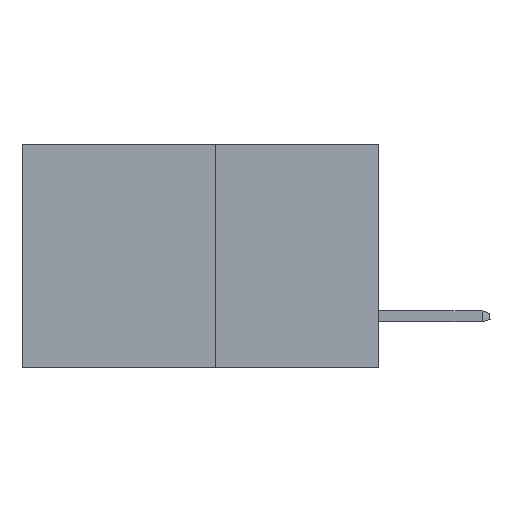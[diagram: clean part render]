
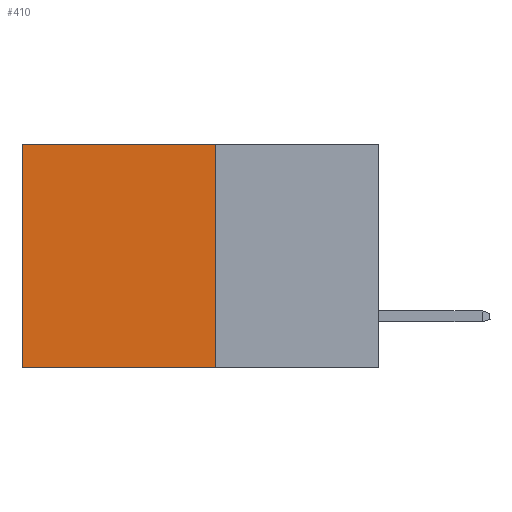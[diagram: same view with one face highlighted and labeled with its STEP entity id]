
A CAD part, left-side view. The second image highlights one B-rep face of the part: STEP entity #410.
In plain terms, the highlighted planar face has unit normal (-1, 0, 0).
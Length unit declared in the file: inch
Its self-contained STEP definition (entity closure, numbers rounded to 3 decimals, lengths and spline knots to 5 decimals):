
#97 = CARTESIAN_POINT ( 'NONE',  ( 0.277, 0.27, -0.37 ) ) ;
#312 = CARTESIAN_POINT ( 'NONE',  ( 0.277, 0.27, 0. ) ) ;
#410 = ADVANCED_FACE ( 'NONE', ( #12683 ), #1009, .F. ) ;
#500 = CARTESIAN_POINT ( 'NONE',  ( 0.277, 0.59, 0. ) ) ;
#1009 = PLANE ( 'NONE',  #9625 ) ;
#1131 = CARTESIAN_POINT ( 'NONE',  ( 0.277, 0.27, -0.37 ) ) ;
#1248 = CARTESIAN_POINT ( 'NONE',  ( 0.277, 0.27, -0.37 ) ) ;
#1303 = DIRECTION ( 'NONE',  ( 0., 0., -1. ) ) ;
#1486 = VECTOR ( 'NONE', #5163, 39.37008 ) ;
#2164 = DIRECTION ( 'NONE',  ( 0., 1., 0. ) ) ;
#3169 = VERTEX_POINT ( 'NONE', #9500 ) ;
#4032 = CARTESIAN_POINT ( 'NONE',  ( 0.277, 0.27, -0.37 ) ) ;
#4869 = LINE ( 'NONE', #1131, #10010 ) ;
#5163 = DIRECTION ( 'NONE',  ( 0., 1., 0. ) ) ;
#5440 = VERTEX_POINT ( 'NONE', #312 ) ;
#5594 = CARTESIAN_POINT ( 'NONE',  ( 0.277, 0.59, -0.37 ) ) ;
#5922 = LINE ( 'NONE', #5594, #8977 ) ;
#6097 = EDGE_CURVE ( 'NONE', #9296, #3169, #4869, .T. ) ;
#7016 = DIRECTION ( 'NONE',  ( 1., 0., 0. ) ) ;
#7064 = LINE ( 'NONE', #1248, #12114 ) ;
#7528 = VERTEX_POINT ( 'NONE', #500 ) ;
#7992 = EDGE_CURVE ( 'NONE', #5440, #9296, #7064, .T. ) ;
#8486 = EDGE_CURVE ( 'NONE', #5440, #7528, #9137, .T. ) ;
#8743 = EDGE_CURVE ( 'NONE', #7528, #3169, #5922, .T. ) ;
#8977 = VECTOR ( 'NONE', #12682, 39.37008 ) ;
#9137 = LINE ( 'NONE', #12258, #1486 ) ;
#9296 = VERTEX_POINT ( 'NONE', #97 ) ;
#9500 = CARTESIAN_POINT ( 'NONE',  ( 0.277, 0.59, -0.37 ) ) ;
#9625 = AXIS2_PLACEMENT_3D ( 'NONE', #4032, #7016, #10243 ) ;
#10010 = VECTOR ( 'NONE', #2164, 39.37008 ) ;
#10243 = DIRECTION ( 'NONE',  ( 0., 0., -1. ) ) ;
#10253 = ORIENTED_EDGE ( 'NONE', *, *, #6097, .F. ) ;
#11364 = ORIENTED_EDGE ( 'NONE', *, *, #8486, .T. ) ;
#12114 = VECTOR ( 'NONE', #1303, 39.37008 ) ;
#12212 = EDGE_LOOP ( 'NONE', ( #12726, #10253, #13310, #11364 ) ) ;
#12258 = CARTESIAN_POINT ( 'NONE',  ( 0.277, 0.27, 0. ) ) ;
#12682 = DIRECTION ( 'NONE',  ( 0., 0., -1. ) ) ;
#12683 = FACE_OUTER_BOUND ( 'NONE', #12212, .T. ) ;
#12726 = ORIENTED_EDGE ( 'NONE', *, *, #8743, .T. ) ;
#13310 = ORIENTED_EDGE ( 'NONE', *, *, #7992, .F. ) ;
